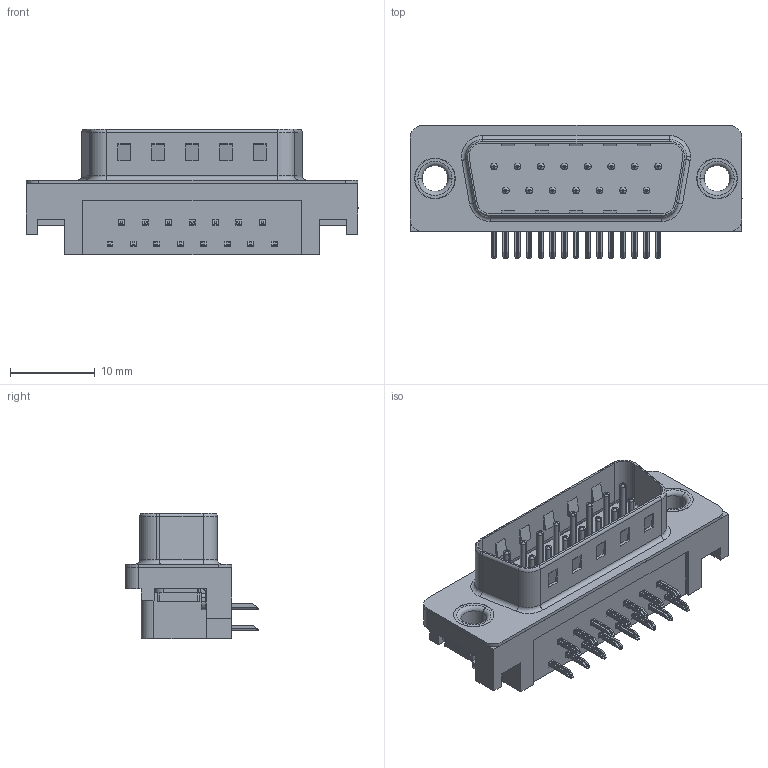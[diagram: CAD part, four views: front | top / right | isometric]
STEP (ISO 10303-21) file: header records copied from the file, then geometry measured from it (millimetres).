
FILE_DESCRIPTION (( 'STEP AP203' ), '1' );
FILE_NAME ('623-015-661-501.STEP', '2018-11-06T12:36:53', ( '' ), ( '' ), 'SwSTEP 2.0', 'SolidWorks 2016', '' );
FILE_SCHEMA (( 'CONFIG_CONTROL_DESIGN' ));
Length unit declared in the file: millimetre
Products named in the file (7): 623 Non Board Mount; 623 Housing_15 Socket; 623-015-661-501; 623 Shell_15 Socket; 623 Thru Hole Rivet; 623 Contact Bottom; 623 Contact Top
Assembly tree (21 placements, depth 2):
  623-015-661-501
    623 Housing_15 Socket
    623 Shell_15 Socket
    623 Contact Bottom  x7
    623 Contact Top  x8
    623 Non Board Mount  x2
    623 Thru Hole Rivet  x2
Bounding box: 39.22 x 15.73 x 14.8 mm (x, y, z)
Volume: 3305.8 mm3; surface area: 4861.2 mm2
Topology: 21 solids, 21 shells, 1427 faces, 3525 edges, 2181 vertices
Faces by surface type: plane 893, cylinder 417, torus 117
Entity records: 16253 total; most frequent: DIRECTION 2680, CARTESIAN_POINT 2625, ORIENTED_EDGE 2520, EDGE_CURVE 1260, AXIS2_PLACEMENT_3D 898, LINE 884, VECTOR 884, VERTEX_POINT 803
